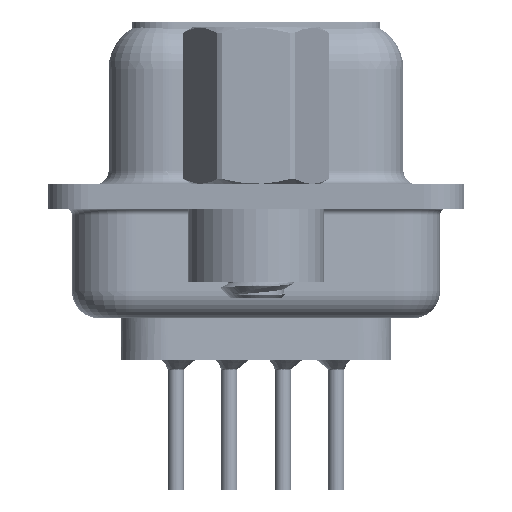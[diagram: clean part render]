
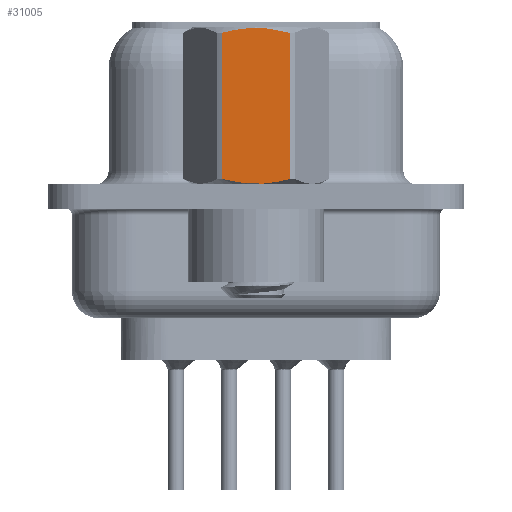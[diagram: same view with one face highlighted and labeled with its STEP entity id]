
A CAD part, left-side view. The second image highlights one B-rep face of the part: STEP entity #31005.
In plain terms, the highlighted planar face has unit normal (-1, 0, 0).
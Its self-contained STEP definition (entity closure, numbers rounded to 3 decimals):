
#40 = CARTESIAN_POINT ( 'NONE',  ( -2.381, -1.273, 6.048 ) ) ;
#82 = CARTESIAN_POINT ( 'NONE',  ( -2.381, -1.066, 0.596 ) ) ;
#614 = DIRECTION ( 'NONE',  ( 0., -1., 0. ) ) ;
#1063 = CARTESIAN_POINT ( 'NONE',  ( -2.381, 1.273, 3.792 ) ) ;
#1439 = CARTESIAN_POINT ( 'NONE',  ( -2.381, -1.273, 0.652 ) ) ;
#1470 = VECTOR ( 'NONE', #15699, 1000. ) ;
#2815 = CARTESIAN_POINT ( 'NONE',  ( -2.381, 1.273, 6.048 ) ) ;
#3966 = ORIENTED_EDGE ( 'NONE', *, *, #28559, .T. ) ;
#5145 = CARTESIAN_POINT ( 'NONE',  ( -2.381, -0.858, 0.55 ) ) ;
#6044 = CARTESIAN_POINT ( 'NONE',  ( -2.381, 0.428, 6.215 ) ) ;
#7252 = ORIENTED_EDGE ( 'NONE', *, *, #27372, .T. ) ;
#7353 = B_SPLINE_CURVE_WITH_KNOTS ( 'NONE', 3,
 ( #57835, #8981, #28654, #28032, #38171, #23608, #24230, #5145, #82, #47995 ),
 .UNSPECIFIED., .F., .F.,
 ( 4, 2, 2, 2, 4 ),
 ( 0.003, 0.003, 0.004, 0.004, 0.005 ),
 .UNSPECIFIED. ) ;
#8981 = CARTESIAN_POINT ( 'NONE',  ( -2.381, 1.065, 0.596 ) ) ;
#9123 = LINE ( 'NONE', #46886, #51187 ) ;
#10148 = FACE_OUTER_BOUND ( 'NONE', #26588, .T. ) ;
#10837 = CARTESIAN_POINT ( 'NONE',  ( -2.381, -0.858, 6.15 ) ) ;
#15699 = DIRECTION ( 'NONE',  ( 0., 0., -1. ) ) ;
#15927 = CARTESIAN_POINT ( 'NONE',  ( -2.381, -0.432, 6.215 ) ) ;
#19448 = CARTESIAN_POINT ( 'NONE',  ( -2.381, 0.853, 6.151 ) ) ;
#23608 = CARTESIAN_POINT ( 'NONE',  ( -2.381, -0.215, 0.468 ) ) ;
#24230 = CARTESIAN_POINT ( 'NONE',  ( -2.381, -0.432, 0.485 ) ) ;
#24509 = CARTESIAN_POINT ( 'NONE',  ( -2.381, 0.215, 6.232 ) ) ;
#25454 = CARTESIAN_POINT ( 'NONE',  ( -2.381, -1.066, 6.104 ) ) ;
#26588 = EDGE_LOOP ( 'NONE', ( #53472, #7252, #3966, #32990 ) ) ;
#26602 = EDGE_CURVE ( 'NONE', #56956, #56411, #44233, .T. ) ;
#27372 = EDGE_CURVE ( 'NONE', #38406, #50262, #9123, .T. ) ;
#28032 = CARTESIAN_POINT ( 'NONE',  ( -2.381, 0.428, 0.485 ) ) ;
#28362 = CARTESIAN_POINT ( 'NONE',  ( -2.381, -1.273, 6.048 ) ) ;
#28559 = EDGE_CURVE ( 'NONE', #50262, #56956, #49308, .T. ) ;
#28654 = CARTESIAN_POINT ( 'NONE',  ( -2.381, 0.853, 0.549 ) ) ;
#31005 = ADVANCED_FACE ( 'NONE', ( #10148 ), #35205, .T. ) ;
#32990 = ORIENTED_EDGE ( 'NONE', *, *, #26602, .T. ) ;
#35205 = PLANE ( 'NONE',  #62544 ) ;
#35684 = EDGE_CURVE ( 'NONE', #56411, #38406, #7353, .T. ) ;
#38171 = CARTESIAN_POINT ( 'NONE',  ( -2.381, 0.215, 0.468 ) ) ;
#38406 = VERTEX_POINT ( 'NONE', #1439 ) ;
#41008 = CARTESIAN_POINT ( 'NONE',  ( -2.381, 1.273, 0.652 ) ) ;
#43839 = CARTESIAN_POINT ( 'NONE',  ( -2.381, 1.273, 6.048 ) ) ;
#44103 = CARTESIAN_POINT ( 'NONE',  ( -2.381, 1.375, -3.75 ) ) ;
#44233 = LINE ( 'NONE', #1063, #1470 ) ;
#46886 = CARTESIAN_POINT ( 'NONE',  ( -2.381, -1.273, 3.792 ) ) ;
#47995 = CARTESIAN_POINT ( 'NONE',  ( -2.381, -1.273, 0.652 ) ) ;
#48569 = CARTESIAN_POINT ( 'NONE',  ( -2.381, 1.065, 6.104 ) ) ;
#49308 = B_SPLINE_CURVE_WITH_KNOTS ( 'NONE', 3,
 ( #40, #25454, #10837, #15927, #53337, #24509, #6044, #19448, #48569, #43839 ),
 .UNSPECIFIED., .F., .F.,
 ( 4, 2, 2, 2, 4 ),
 ( 0.001, 0.002, 0.002, 0.003, 0.004 ),
 .UNSPECIFIED. ) ;
#50262 = VERTEX_POINT ( 'NONE', #28362 ) ;
#51187 = VECTOR ( 'NONE', #62414, 1000. ) ;
#53337 = CARTESIAN_POINT ( 'NONE',  ( -2.381, -0.215, 6.232 ) ) ;
#53472 = ORIENTED_EDGE ( 'NONE', *, *, #35684, .T. ) ;
#54557 = DIRECTION ( 'NONE',  ( -1., 0., 0. ) ) ;
#56411 = VERTEX_POINT ( 'NONE', #41008 ) ;
#56956 = VERTEX_POINT ( 'NONE', #2815 ) ;
#57835 = CARTESIAN_POINT ( 'NONE',  ( -2.381, 1.273, 0.652 ) ) ;
#62414 = DIRECTION ( 'NONE',  ( 0., 0., 1. ) ) ;
#62544 = AXIS2_PLACEMENT_3D ( 'NONE', #44103, #54557, #614 ) ;
